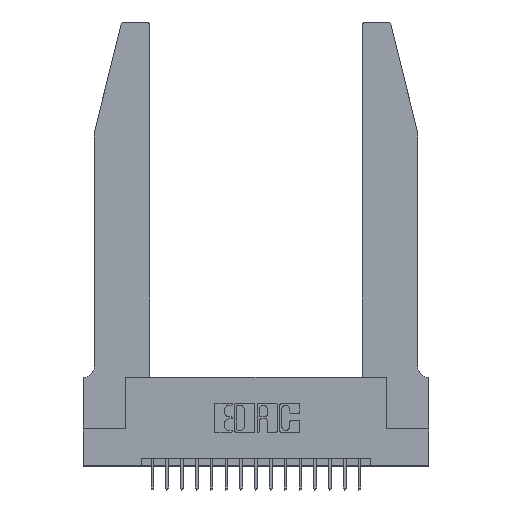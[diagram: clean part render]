
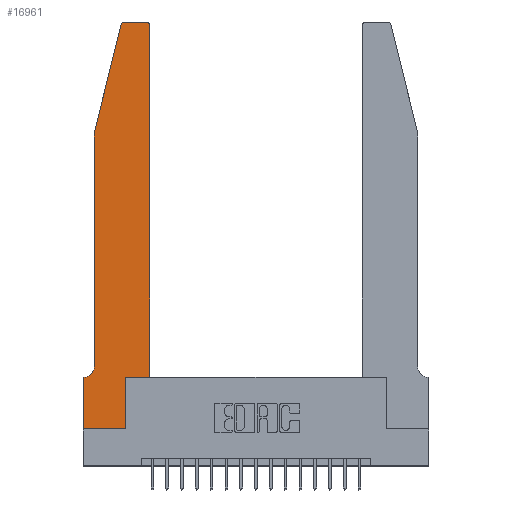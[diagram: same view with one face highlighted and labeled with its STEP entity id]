
A CAD part, top view. The second image highlights one B-rep face of the part: STEP entity #16961.
In plain terms, the highlighted planar face has unit normal (0, 0, 1).
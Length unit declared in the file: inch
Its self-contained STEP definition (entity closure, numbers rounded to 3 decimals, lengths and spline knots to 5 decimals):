
#50 = EDGE_CURVE ( 'NONE', #19653, #10282, #12421, .T. ) ;
#224 = CARTESIAN_POINT ( 'NONE',  ( 0.4205, 2.72, 0.37 ) ) ;
#633 = EDGE_CURVE ( 'NONE', #10282, #20216, #13013, .T. ) ;
#1793 = DIRECTION ( 'NONE',  ( 1., 0., 0. ) ) ;
#2239 = VERTEX_POINT ( 'NONE', #19075 ) ;
#2255 = EDGE_CURVE ( 'NONE', #4785, #10165, #15090, .T. ) ;
#2628 = ORIENTED_EDGE ( 'NONE', *, *, #17283, .T. ) ;
#2676 = CARTESIAN_POINT ( 'NONE',  ( 0.2865, 0.35, 0.37 ) ) ;
#2799 = LINE ( 'NONE', #11202, #14746 ) ;
#2892 = VECTOR ( 'NONE', #18419, 39.37008 ) ;
#3367 = LINE ( 'NONE', #4308, #19284 ) ;
#3470 = EDGE_CURVE ( 'NONE', #19505, #10511, #7840, .T. ) ;
#3705 = VECTOR ( 'NONE', #12870, 39.37008 ) ;
#3732 = ORIENTED_EDGE ( 'NONE', *, *, #17898, .T. ) ;
#3922 = LINE ( 'NONE', #6151, #2892 ) ;
#4308 = CARTESIAN_POINT ( 'NONE',  ( 0.0755, 2., 0.37 ) ) ;
#4323 = VECTOR ( 'NONE', #1793, 39.37008 ) ;
#4746 = VECTOR ( 'NONE', #18084, 39.37008 ) ;
#4785 = VERTEX_POINT ( 'NONE', #16735 ) ;
#4912 = ORIENTED_EDGE ( 'NONE', *, *, #7643, .T. ) ;
#5246 = LINE ( 'NONE', #19554, #4746 ) ;
#5285 = CARTESIAN_POINT ( 'NONE',  ( 0.284, 2.72, 0.37 ) ) ;
#5537 = CARTESIAN_POINT ( 'NONE',  ( 0.0755, 0.35, 0.37 ) ) ;
#6017 = ORIENTED_EDGE ( 'NONE', *, *, #8974, .T. ) ;
#6138 = CARTESIAN_POINT ( 'NONE',  ( 0.0055, 0.42, 0.37 ) ) ;
#6149 = EDGE_CURVE ( 'NONE', #15649, #2239, #12594, .T. ) ;
#6151 = CARTESIAN_POINT ( 'NONE',  ( 0.2605, 2.75, 0.37 ) ) ;
#6287 = ORIENTED_EDGE ( 'NONE', *, *, #2255, .T. ) ;
#6370 = ORIENTED_EDGE ( 'NONE', *, *, #3470, .T. ) ;
#6569 = LINE ( 'NONE', #5537, #10230 ) ;
#6690 = DIRECTION ( 'NONE',  ( 0., 0., -1. ) ) ;
#6843 = DIRECTION ( 'NONE',  ( 1., 0., 0. ) ) ;
#7098 = DIRECTION ( 'NONE',  ( -1., 0., 0. ) ) ;
#7262 = DIRECTION ( 'NONE',  ( 1., 0., 0. ) ) ;
#7394 = CARTESIAN_POINT ( 'NONE',  ( 0.2865, 0.35, 0.37 ) ) ;
#7643 = EDGE_CURVE ( 'NONE', #15118, #15649, #12616, .T. ) ;
#7840 = CIRCLE ( 'NONE', #13647, 0.03 ) ;
#7843 = ORIENTED_EDGE ( 'NONE', *, *, #12883, .T. ) ;
#8137 = CARTESIAN_POINT ( 'NONE',  ( 0.4505, 0.35, 0.37 ) ) ;
#8156 = DIRECTION ( 'NONE',  ( 0., 0., 1. ) ) ;
#8176 = VERTEX_POINT ( 'NONE', #11927 ) ;
#8254 = CARTESIAN_POINT ( 'NONE',  ( 0., 0., 0.37 ) ) ;
#8440 = DIRECTION ( 'NONE',  ( -1., 0., 0. ) ) ;
#8802 = CARTESIAN_POINT ( 'NONE',  ( 0.0755, 2., 0.37 ) ) ;
#8974 = EDGE_CURVE ( 'NONE', #2239, #19505, #2799, .T. ) ;
#8986 = VECTOR ( 'NONE', #18113, 39.37008 ) ;
#9014 = DIRECTION ( 'NONE',  ( -0.239, -0.971, 0. ) ) ;
#9126 = ORIENTED_EDGE ( 'NONE', *, *, #6149, .T. ) ;
#9603 = ORIENTED_EDGE ( 'NONE', *, *, #10647, .T. ) ;
#9741 = EDGE_LOOP ( 'NONE', ( #7843, #2628, #10950, #20126, #16736, #3732, #6287, #9603, #4912, #9126, #6017, #6370 ) ) ;
#9997 = FACE_OUTER_BOUND ( 'NONE', #9741, .T. ) ;
#10071 = DIRECTION ( 'NONE',  ( 0., -1., 0. ) ) ;
#10165 = VERTEX_POINT ( 'NONE', #16846 ) ;
#10230 = VECTOR ( 'NONE', #7098, 39.37008 ) ;
#10282 = VERTEX_POINT ( 'NONE', #14197 ) ;
#10313 = PLANE ( 'NONE',  #17667 ) ;
#10511 = VERTEX_POINT ( 'NONE', #19363 ) ;
#10647 = EDGE_CURVE ( 'NONE', #10165, #15118, #5246, .T. ) ;
#10950 = ORIENTED_EDGE ( 'NONE', *, *, #17546, .T. ) ;
#11202 = CARTESIAN_POINT ( 'NONE',  ( 0.4505, 0.35, 0.37 ) ) ;
#11575 = CARTESIAN_POINT ( 'NONE',  ( 0.4505, 2.72, 0.37 ) ) ;
#11927 = CARTESIAN_POINT ( 'NONE',  ( 0.25487, 2.72718, 0.37 ) ) ;
#11937 = CIRCLE ( 'NONE', #18285, 0.03 ) ;
#12421 = LINE ( 'NONE', #15458, #15974 ) ;
#12594 = LINE ( 'NONE', #8137, #4323 ) ;
#12616 = LINE ( 'NONE', #7394, #8986 ) ;
#12765 = DIRECTION ( 'NONE',  ( 0., 1., 0. ) ) ;
#12870 = DIRECTION ( 'NONE',  ( 0., -1., 0. ) ) ;
#12883 = EDGE_CURVE ( 'NONE', #10511, #19826, #3922, .T. ) ;
#13013 = CIRCLE ( 'NONE', #18664, 0.07 ) ;
#13647 = AXIS2_PLACEMENT_3D ( 'NONE', #224, #8156, #20191 ) ;
#14197 = CARTESIAN_POINT ( 'NONE',  ( 0.0755, 0.42, 0.37 ) ) ;
#14746 = VECTOR ( 'NONE', #12765, 39.37008 ) ;
#15090 = LINE ( 'NONE', #8254, #3705 ) ;
#15118 = VERTEX_POINT ( 'NONE', #18049 ) ;
#15458 = CARTESIAN_POINT ( 'NONE',  ( 0.0755, 2., 0.37 ) ) ;
#15649 = VERTEX_POINT ( 'NONE', #2676 ) ;
#15974 = VECTOR ( 'NONE', #10071, 39.37008 ) ;
#16059 = DIRECTION ( 'NONE',  ( 0., 0., 1. ) ) ;
#16218 = CARTESIAN_POINT ( 'NONE',  ( 0.0055, 0.35, 0.37 ) ) ;
#16481 = DIRECTION ( 'NONE',  ( 0., 0., 1. ) ) ;
#16735 = CARTESIAN_POINT ( 'NONE',  ( 0., 0.35, 0.37 ) ) ;
#16736 = ORIENTED_EDGE ( 'NONE', *, *, #633, .T. ) ;
#16820 = CARTESIAN_POINT ( 'NONE',  ( 0.284, 2.75, 0.37 ) ) ;
#16846 = CARTESIAN_POINT ( 'NONE',  ( 0., 0., 0.37 ) ) ;
#16961 = ADVANCED_FACE ( 'NONE', ( #9997 ), #10313, .T. ) ;
#17283 = EDGE_CURVE ( 'NONE', #19826, #8176, #11937, .T. ) ;
#17546 = EDGE_CURVE ( 'NONE', #8176, #19653, #3367, .T. ) ;
#17667 = AXIS2_PLACEMENT_3D ( 'NONE', #19450, #16481, #7262 ) ;
#17898 = EDGE_CURVE ( 'NONE', #20216, #4785, #6569, .T. ) ;
#18049 = CARTESIAN_POINT ( 'NONE',  ( 0.2865, 0., 0.37 ) ) ;
#18084 = DIRECTION ( 'NONE',  ( 1., 0., 0. ) ) ;
#18113 = DIRECTION ( 'NONE',  ( 0., 1., 0. ) ) ;
#18285 = AXIS2_PLACEMENT_3D ( 'NONE', #5285, #16059, #6843 ) ;
#18419 = DIRECTION ( 'NONE',  ( -1., 0., 0. ) ) ;
#18664 = AXIS2_PLACEMENT_3D ( 'NONE', #6138, #6690, #8440 ) ;
#19075 = CARTESIAN_POINT ( 'NONE',  ( 0.4505, 0.35, 0.37 ) ) ;
#19284 = VECTOR ( 'NONE', #9014, 39.37008 ) ;
#19363 = CARTESIAN_POINT ( 'NONE',  ( 0.4205, 2.75, 0.37 ) ) ;
#19450 = CARTESIAN_POINT ( 'NONE',  ( 0., 0.35, 0.37 ) ) ;
#19505 = VERTEX_POINT ( 'NONE', #11575 ) ;
#19554 = CARTESIAN_POINT ( 'NONE',  ( 0., 0., 0.37 ) ) ;
#19653 = VERTEX_POINT ( 'NONE', #8802 ) ;
#19826 = VERTEX_POINT ( 'NONE', #16820 ) ;
#20126 = ORIENTED_EDGE ( 'NONE', *, *, #50, .T. ) ;
#20191 = DIRECTION ( 'NONE',  ( 1., 0., 0. ) ) ;
#20216 = VERTEX_POINT ( 'NONE', #16218 ) ;
